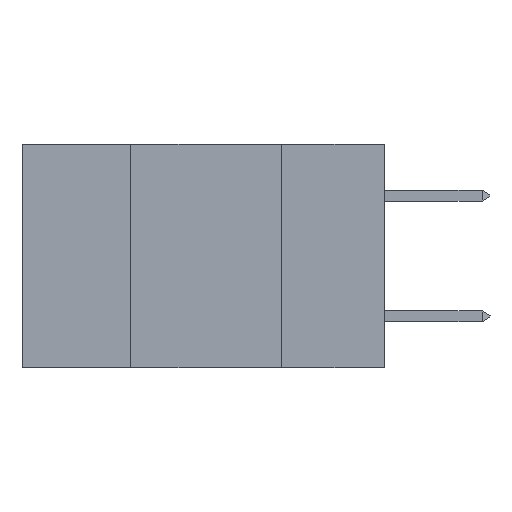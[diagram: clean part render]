
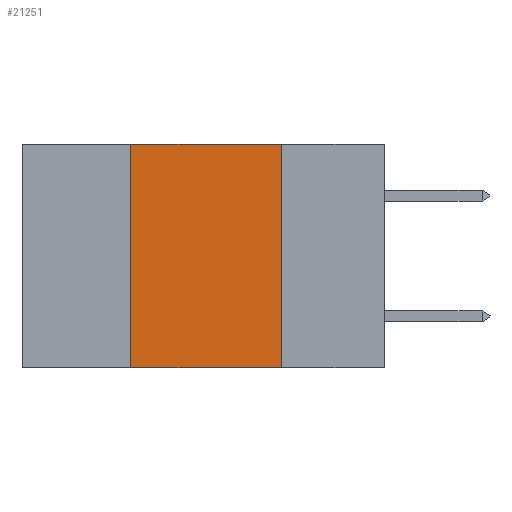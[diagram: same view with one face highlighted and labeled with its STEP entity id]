
A CAD part, left-side view. The second image highlights one B-rep face of the part: STEP entity #21251.
In plain terms, the highlighted planar face has unit normal (-1, 0, 0).
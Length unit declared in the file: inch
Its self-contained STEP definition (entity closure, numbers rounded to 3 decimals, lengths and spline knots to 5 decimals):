
#2386 = DIRECTION ( 'NONE',  ( 0., 0., -1. ) ) ;
#4287 = ORIENTED_EDGE ( 'NONE', *, *, #10153, .F. ) ;
#5062 = PLANE ( 'NONE',  #15469 ) ;
#5206 = CARTESIAN_POINT ( 'NONE',  ( 0., 0.17, 0. ) ) ;
#5430 = DIRECTION ( 'NONE',  ( 1., 0., 0. ) ) ;
#5981 = VERTEX_POINT ( 'NONE', #16813 ) ;
#6691 = EDGE_CURVE ( 'NONE', #5981, #6917, #10320, .T. ) ;
#6747 = CARTESIAN_POINT ( 'NONE',  ( 0., 0.17, 0. ) ) ;
#6917 = VERTEX_POINT ( 'NONE', #6747 ) ;
#9332 = EDGE_LOOP ( 'NONE', ( #4287, #12104, #10423, #18205 ) ) ;
#9386 = VECTOR ( 'NONE', #24492, 39.37008 ) ;
#10134 = CARTESIAN_POINT ( 'NONE',  ( 0., 0.6, 0. ) ) ;
#10153 = EDGE_CURVE ( 'NONE', #6917, #11413, #30773, .T. ) ;
#10320 = LINE ( 'NONE', #10134, #9386 ) ;
#10423 = ORIENTED_EDGE ( 'NONE', *, *, #17671, .F. ) ;
#10850 = DIRECTION ( 'NONE',  ( 0., 0., -1. ) ) ;
#11413 = VERTEX_POINT ( 'NONE', #28770 ) ;
#12104 = ORIENTED_EDGE ( 'NONE', *, *, #6691, .F. ) ;
#13210 = VERTEX_POINT ( 'NONE', #22442 ) ;
#15249 = LINE ( 'NONE', #35206, #35508 ) ;
#15469 = AXIS2_PLACEMENT_3D ( 'NONE', #33055, #5430, #10850 ) ;
#16813 = CARTESIAN_POINT ( 'NONE',  ( 0., 0.42, 0. ) ) ;
#17319 = LINE ( 'NONE', #20299, #29656 ) ;
#17498 = DIRECTION ( 'NONE',  ( 0., 0., 1. ) ) ;
#17671 = EDGE_CURVE ( 'NONE', #13210, #5981, #17319, .T. ) ;
#18205 = ORIENTED_EDGE ( 'NONE', *, *, #24167, .T. ) ;
#19228 = VECTOR ( 'NONE', #2386, 39.37008 ) ;
#20299 = CARTESIAN_POINT ( 'NONE',  ( 0., 0.42, 0. ) ) ;
#21251 = ADVANCED_FACE ( 'NONE', ( #22222 ), #5062, .F. ) ;
#22222 = FACE_OUTER_BOUND ( 'NONE', #9332, .T. ) ;
#22442 = CARTESIAN_POINT ( 'NONE',  ( 0., 0.42, -0.37 ) ) ;
#24167 = EDGE_CURVE ( 'NONE', #13210, #11413, #15249, .T. ) ;
#24492 = DIRECTION ( 'NONE',  ( 0., -1., 0. ) ) ;
#26621 = DIRECTION ( 'NONE',  ( 0., -1., 0. ) ) ;
#28770 = CARTESIAN_POINT ( 'NONE',  ( 0., 0.17, -0.37 ) ) ;
#29656 = VECTOR ( 'NONE', #17498, 39.37008 ) ;
#30773 = LINE ( 'NONE', #5206, #19228 ) ;
#33055 = CARTESIAN_POINT ( 'NONE',  ( 0., 0.6, 0. ) ) ;
#35206 = CARTESIAN_POINT ( 'NONE',  ( 0., 0.6, -0.37 ) ) ;
#35508 = VECTOR ( 'NONE', #26621, 39.37008 ) ;
